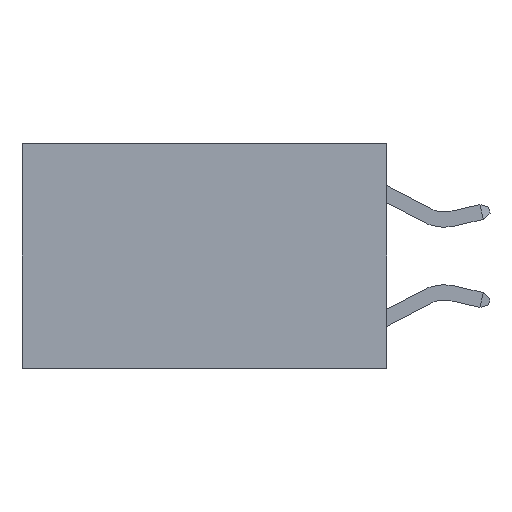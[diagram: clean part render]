
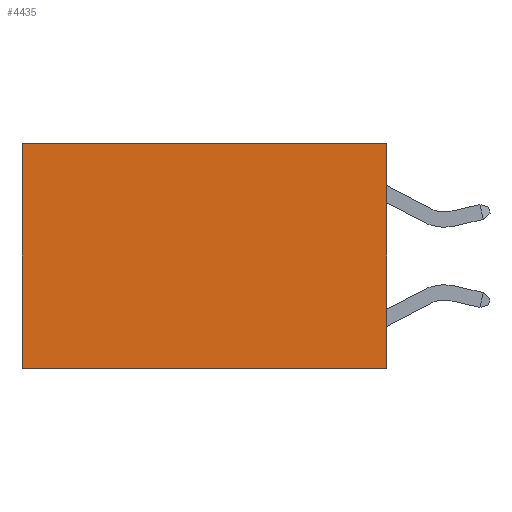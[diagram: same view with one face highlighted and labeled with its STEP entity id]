
A CAD part, left-side view. The second image highlights one B-rep face of the part: STEP entity #4435.
In plain terms, the highlighted planar face has unit normal (-1, 0, 0).
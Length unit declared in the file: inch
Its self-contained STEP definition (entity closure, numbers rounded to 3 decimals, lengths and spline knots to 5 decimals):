
#59 = CARTESIAN_POINT ( 'NONE',  ( 0.2625, 0., 0. ) ) ;
#999 = LINE ( 'NONE', #1256, #3171 ) ;
#1002 = AXIS2_PLACEMENT_3D ( 'NONE', #7339, #7951, #6857 ) ;
#1256 = CARTESIAN_POINT ( 'NONE',  ( 0.2625, 0., 0. ) ) ;
#1387 = LINE ( 'NONE', #59, #4751 ) ;
#1704 = VECTOR ( 'NONE', #7012, 39.37008 ) ;
#2043 = CARTESIAN_POINT ( 'NONE',  ( 0.2625, 0., -0.37 ) ) ;
#2135 = LINE ( 'NONE', #7251, #5177 ) ;
#3171 = VECTOR ( 'NONE', #5027, 39.37008 ) ;
#3242 = CARTESIAN_POINT ( 'NONE',  ( 0.2625, 0., -0.37 ) ) ;
#3244 = DIRECTION ( 'NONE',  ( 0., 1., 0. ) ) ;
#3265 = VERTEX_POINT ( 'NONE', #2043 ) ;
#3378 = LINE ( 'NONE', #3242, #1704 ) ;
#3400 = VERTEX_POINT ( 'NONE', #5307 ) ;
#3714 = ORIENTED_EDGE ( 'NONE', *, *, #7197, .T. ) ;
#3800 = VERTEX_POINT ( 'NONE', #8182 ) ;
#4428 = EDGE_LOOP ( 'NONE', ( #7939, #7651, #5182, #3714 ) ) ;
#4435 = ADVANCED_FACE ( 'NONE', ( #5514 ), #6047, .F. ) ;
#4751 = VECTOR ( 'NONE', #3244, 39.37008 ) ;
#5027 = DIRECTION ( 'NONE',  ( 0., 0., -1. ) ) ;
#5177 = VECTOR ( 'NONE', #6602, 39.37008 ) ;
#5182 = ORIENTED_EDGE ( 'NONE', *, *, #7640, .F. ) ;
#5307 = CARTESIAN_POINT ( 'NONE',  ( 0.2625, 0.6, -0.37 ) ) ;
#5514 = FACE_OUTER_BOUND ( 'NONE', #4428, .T. ) ;
#6047 = PLANE ( 'NONE',  #1002 ) ;
#6602 = DIRECTION ( 'NONE',  ( 0., 0., -1. ) ) ;
#6857 = DIRECTION ( 'NONE',  ( 0., 0., -1. ) ) ;
#6912 = EDGE_CURVE ( 'NONE', #3265, #3400, #3378, .T. ) ;
#6983 = VERTEX_POINT ( 'NONE', #7699 ) ;
#7012 = DIRECTION ( 'NONE',  ( 0., 1., 0. ) ) ;
#7197 = EDGE_CURVE ( 'NONE', #3800, #6983, #1387, .T. ) ;
#7251 = CARTESIAN_POINT ( 'NONE',  ( 0.2625, 0.6, 0. ) ) ;
#7339 = CARTESIAN_POINT ( 'NONE',  ( 0.2625, 0., 0. ) ) ;
#7640 = EDGE_CURVE ( 'NONE', #3800, #3265, #999, .T. ) ;
#7651 = ORIENTED_EDGE ( 'NONE', *, *, #6912, .F. ) ;
#7699 = CARTESIAN_POINT ( 'NONE',  ( 0.2625, 0.6, 0. ) ) ;
#7865 = EDGE_CURVE ( 'NONE', #6983, #3400, #2135, .T. ) ;
#7939 = ORIENTED_EDGE ( 'NONE', *, *, #7865, .T. ) ;
#7951 = DIRECTION ( 'NONE',  ( 1., 0., 0. ) ) ;
#8182 = CARTESIAN_POINT ( 'NONE',  ( 0.2625, 0., 0. ) ) ;
